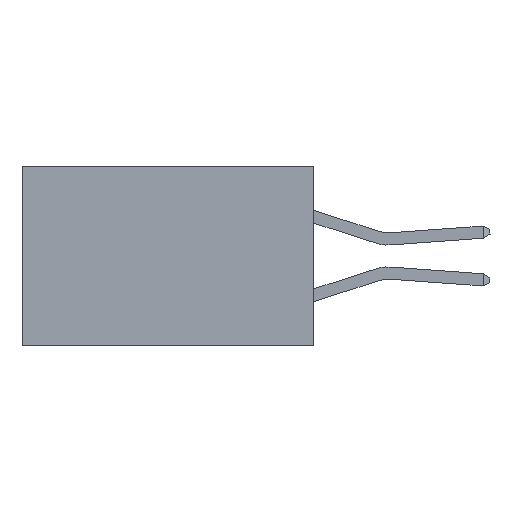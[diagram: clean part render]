
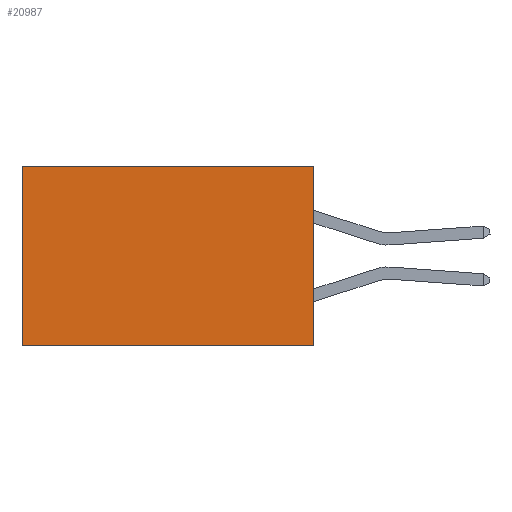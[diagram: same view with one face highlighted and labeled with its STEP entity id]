
A CAD part, left-side view. The second image highlights one B-rep face of the part: STEP entity #20987.
In plain terms, the highlighted planar face has unit normal (-1, 0, 0).
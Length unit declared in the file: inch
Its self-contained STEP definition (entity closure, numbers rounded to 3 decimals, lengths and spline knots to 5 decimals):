
#1201 = EDGE_LOOP ( 'NONE', ( #9162, #9089, #10594, #22630 ) ) ;
#1492 = DIRECTION ( 'NONE',  ( 0., 1., 0. ) ) ;
#1544 = CARTESIAN_POINT ( 'NONE',  ( 0.2875, 0.6, 0. ) ) ;
#1713 = DIRECTION ( 'NONE',  ( 0., 0., -1. ) ) ;
#2473 = EDGE_CURVE ( 'NONE', #9837, #10725, #11165, .T. ) ;
#2874 = EDGE_CURVE ( 'NONE', #12654, #10725, #17926, .T. ) ;
#3146 = FACE_OUTER_BOUND ( 'NONE', #1201, .T. ) ;
#3323 = CARTESIAN_POINT ( 'NONE',  ( 0.2875, 0., 0. ) ) ;
#4623 = PLANE ( 'NONE',  #6845 ) ;
#6477 = CARTESIAN_POINT ( 'NONE',  ( 0.2875, 0., -0.37 ) ) ;
#6845 = AXIS2_PLACEMENT_3D ( 'NONE', #8468, #21528, #10381 ) ;
#6925 = CARTESIAN_POINT ( 'NONE',  ( 0.2875, 0.6, 0. ) ) ;
#8468 = CARTESIAN_POINT ( 'NONE',  ( 0.2875, 0., 0. ) ) ;
#8959 = LINE ( 'NONE', #3323, #18373 ) ;
#9089 = ORIENTED_EDGE ( 'NONE', *, *, #2874, .F. ) ;
#9162 = ORIENTED_EDGE ( 'NONE', *, *, #2473, .T. ) ;
#9837 = VERTEX_POINT ( 'NONE', #1544 ) ;
#9872 = EDGE_CURVE ( 'NONE', #14985, #12654, #11435, .T. ) ;
#10381 = DIRECTION ( 'NONE',  ( 0., 0., -1. ) ) ;
#10594 = ORIENTED_EDGE ( 'NONE', *, *, #9872, .F. ) ;
#10725 = VERTEX_POINT ( 'NONE', #11771 ) ;
#10832 = VECTOR ( 'NONE', #1713, 39.37008 ) ;
#11165 = LINE ( 'NONE', #6925, #21065 ) ;
#11435 = LINE ( 'NONE', #24129, #10832 ) ;
#11723 = DIRECTION ( 'NONE',  ( 0., 0., -1. ) ) ;
#11771 = CARTESIAN_POINT ( 'NONE',  ( 0.2875, 0.6, -0.37 ) ) ;
#12215 = DIRECTION ( 'NONE',  ( 0., 1., 0. ) ) ;
#12654 = VERTEX_POINT ( 'NONE', #13565 ) ;
#13565 = CARTESIAN_POINT ( 'NONE',  ( 0.2875, 0., -0.37 ) ) ;
#14985 = VERTEX_POINT ( 'NONE', #22113 ) ;
#16783 = VECTOR ( 'NONE', #12215, 39.37008 ) ;
#17926 = LINE ( 'NONE', #6477, #16783 ) ;
#18373 = VECTOR ( 'NONE', #1492, 39.37008 ) ;
#18466 = EDGE_CURVE ( 'NONE', #14985, #9837, #8959, .T. ) ;
#20987 = ADVANCED_FACE ( 'NONE', ( #3146 ), #4623, .F. ) ;
#21065 = VECTOR ( 'NONE', #11723, 39.37008 ) ;
#21528 = DIRECTION ( 'NONE',  ( 1., 0., 0. ) ) ;
#22113 = CARTESIAN_POINT ( 'NONE',  ( 0.2875, 0., 0. ) ) ;
#22630 = ORIENTED_EDGE ( 'NONE', *, *, #18466, .T. ) ;
#24129 = CARTESIAN_POINT ( 'NONE',  ( 0.2875, 0., 0. ) ) ;
